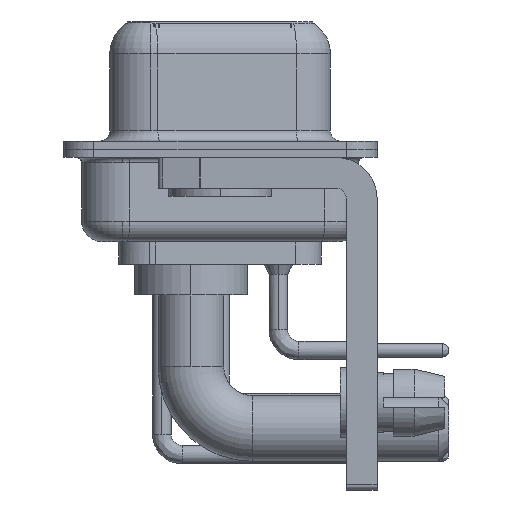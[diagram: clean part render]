
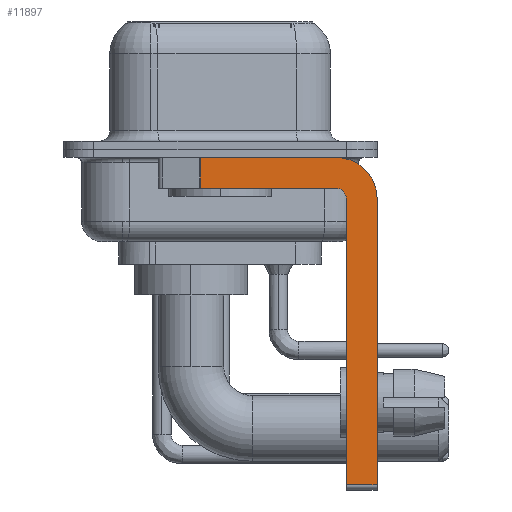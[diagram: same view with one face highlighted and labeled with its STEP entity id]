
A CAD part, left-side view. The second image highlights one B-rep face of the part: STEP entity #11897.
In plain terms, the highlighted planar face has unit normal (-1, 0, 0).
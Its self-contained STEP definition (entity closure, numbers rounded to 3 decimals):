
#177 = CARTESIAN_POINT ( 'NONE',  ( -2.9, -5.65, -0.4 ) ) ;
#545 = CARTESIAN_POINT ( 'NONE',  ( -2.9, -6.15, -16.35 ) ) ;
#1298 = PLANE ( 'NONE',  #2295 ) ;
#1629 = LINE ( 'NONE', #18807, #20922 ) ;
#2218 = LINE ( 'NONE', #21807, #29016 ) ;
#2295 = AXIS2_PLACEMENT_3D ( 'NONE', #13208, #8361, #6423 ) ;
#3403 = VERTEX_POINT ( 'NONE', #22849 ) ;
#3950 = DIRECTION ( 'NONE',  ( -1., 0., 0. ) ) ;
#4996 = EDGE_CURVE ( 'NONE', #3403, #22631, #7228, .T. ) ;
#5894 = LINE ( 'NONE', #8608, #16756 ) ;
#6423 = DIRECTION ( 'NONE',  ( 0., 0., -1. ) ) ;
#6872 = CARTESIAN_POINT ( 'NONE',  ( -2.9, 0.978, -1.9 ) ) ;
#6882 = ORIENTED_EDGE ( 'NONE', *, *, #27072, .F. ) ;
#7228 = LINE ( 'NONE', #31312, #13618 ) ;
#8022 = EDGE_CURVE ( 'NONE', #19485, #18039, #16403, .T. ) ;
#8361 = DIRECTION ( 'NONE',  ( 1., 0., 0. ) ) ;
#8608 = CARTESIAN_POINT ( 'NONE',  ( -2.9, -7.65, -2.4 ) ) ;
#8643 = LINE ( 'NONE', #23410, #27931 ) ;
#11897 = ADVANCED_FACE ( 'NONE', ( #30806 ), #1298, .F. ) ;
#12263 = EDGE_CURVE ( 'NONE', #3403, #30378, #8643, .T. ) ;
#13208 = CARTESIAN_POINT ( 'NONE',  ( -2.9, -5.65, -2.4 ) ) ;
#13618 = VECTOR ( 'NONE', #31156, 1000. ) ;
#13985 = CARTESIAN_POINT ( 'NONE',  ( -2.9, -5.65, -16.35 ) ) ;
#14072 = DIRECTION ( 'NONE',  ( 1., 0., 0. ) ) ;
#14169 = ORIENTED_EDGE ( 'NONE', *, *, #28840, .F. ) ;
#14893 = ORIENTED_EDGE ( 'NONE', *, *, #12263, .T. ) ;
#16112 = ORIENTED_EDGE ( 'NONE', *, *, #21458, .F. ) ;
#16172 = CARTESIAN_POINT ( 'NONE',  ( -2.9, -5.65, -2.4 ) ) ;
#16306 = ORIENTED_EDGE ( 'NONE', *, *, #4996, .F. ) ;
#16403 = LINE ( 'NONE', #13985, #23456 ) ;
#16584 = DIRECTION ( 'NONE',  ( 0., 0., 1. ) ) ;
#16592 = AXIS2_PLACEMENT_3D ( 'NONE', #18869, #14072, #26249 ) ;
#16633 = EDGE_CURVE ( 'NONE', #19485, #23427, #1629, .T. ) ;
#16756 = VECTOR ( 'NONE', #17943, 1000. ) ;
#17695 = EDGE_LOOP ( 'NONE', ( #16306, #14893, #14169, #27396, #24433, #30841, #6882, #16112 ) ) ;
#17943 = DIRECTION ( 'NONE',  ( 0., 0., -1. ) ) ;
#18039 = VERTEX_POINT ( 'NONE', #27713 ) ;
#18717 = EDGE_CURVE ( 'NONE', #23427, #30839, #18889, .T. ) ;
#18807 = CARTESIAN_POINT ( 'NONE',  ( -2.9, -6.15, -16.6 ) ) ;
#18869 = CARTESIAN_POINT ( 'NONE',  ( -2.9, -5.65, -2.4 ) ) ;
#18889 = CIRCLE ( 'NONE', #21470, 0.5 ) ;
#19485 = VERTEX_POINT ( 'NONE', #545 ) ;
#20370 = CARTESIAN_POINT ( 'NONE',  ( -2.9, -7.65, -2.4 ) ) ;
#20922 = VECTOR ( 'NONE', #16584, 1000. ) ;
#21300 = CARTESIAN_POINT ( 'NONE',  ( -2.9, -6.15, -2.4 ) ) ;
#21458 = EDGE_CURVE ( 'NONE', #22631, #24747, #22732, .T. ) ;
#21470 = AXIS2_PLACEMENT_3D ( 'NONE', #16172, #3950, #23543 ) ;
#21807 = CARTESIAN_POINT ( 'NONE',  ( -2.9, -5.65, -1.9 ) ) ;
#22631 = VERTEX_POINT ( 'NONE', #177 ) ;
#22732 = CIRCLE ( 'NONE', #16592, 2. ) ;
#22849 = CARTESIAN_POINT ( 'NONE',  ( -2.9, 0.978, -0.4 ) ) ;
#23410 = CARTESIAN_POINT ( 'NONE',  ( -2.9, 0.978, -1.9 ) ) ;
#23427 = VERTEX_POINT ( 'NONE', #21300 ) ;
#23456 = VECTOR ( 'NONE', #23773, 1000. ) ;
#23543 = DIRECTION ( 'NONE',  ( 0., 0., 1. ) ) ;
#23773 = DIRECTION ( 'NONE',  ( 0., -1., 0. ) ) ;
#24433 = ORIENTED_EDGE ( 'NONE', *, *, #16633, .F. ) ;
#24747 = VERTEX_POINT ( 'NONE', #20370 ) ;
#26249 = DIRECTION ( 'NONE',  ( 0., 0., -1. ) ) ;
#26262 = CARTESIAN_POINT ( 'NONE',  ( -2.9, -5.65, -1.9 ) ) ;
#27072 = EDGE_CURVE ( 'NONE', #24747, #18039, #5894, .T. ) ;
#27396 = ORIENTED_EDGE ( 'NONE', *, *, #18717, .F. ) ;
#27713 = CARTESIAN_POINT ( 'NONE',  ( -2.9, -7.65, -16.35 ) ) ;
#27931 = VECTOR ( 'NONE', #28059, 1000. ) ;
#28059 = DIRECTION ( 'NONE',  ( 0., 0., -1. ) ) ;
#28840 = EDGE_CURVE ( 'NONE', #30839, #30378, #2218, .T. ) ;
#29016 = VECTOR ( 'NONE', #31585, 1000. ) ;
#30378 = VERTEX_POINT ( 'NONE', #6872 ) ;
#30806 = FACE_OUTER_BOUND ( 'NONE', #17695, .T. ) ;
#30839 = VERTEX_POINT ( 'NONE', #26262 ) ;
#30841 = ORIENTED_EDGE ( 'NONE', *, *, #8022, .T. ) ;
#31156 = DIRECTION ( 'NONE',  ( 0., -1., 0. ) ) ;
#31312 = CARTESIAN_POINT ( 'NONE',  ( -2.9, 3., -0.4 ) ) ;
#31585 = DIRECTION ( 'NONE',  ( 0., 1., 0. ) ) ;
